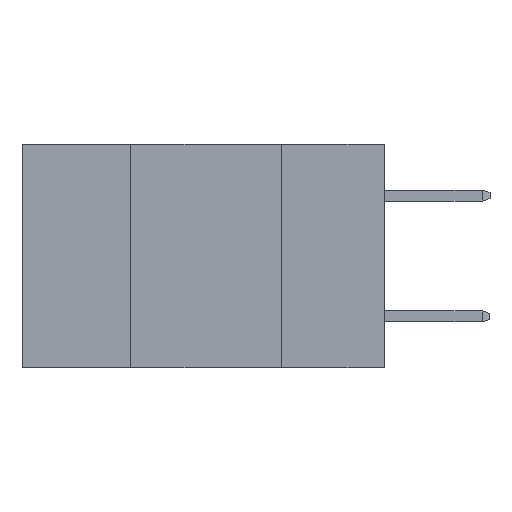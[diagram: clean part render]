
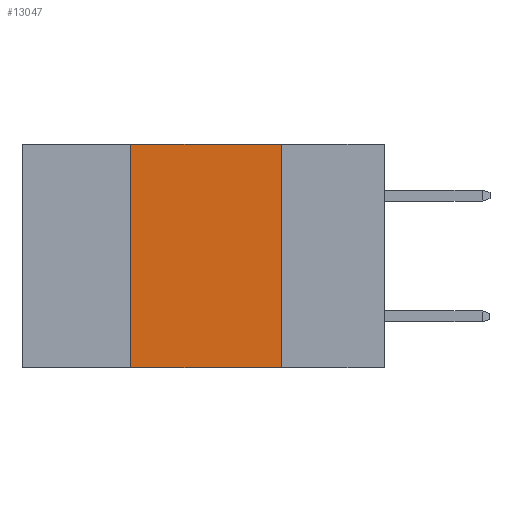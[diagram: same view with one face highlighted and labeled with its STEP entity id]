
A CAD part, left-side view. The second image highlights one B-rep face of the part: STEP entity #13047.
In plain terms, the highlighted planar face has unit normal (-1, 0, 0).
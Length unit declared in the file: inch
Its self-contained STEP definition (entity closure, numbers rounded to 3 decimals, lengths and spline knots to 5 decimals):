
#382 = ORIENTED_EDGE ( 'NONE', *, *, #14201, .F. ) ;
#405 = PLANE ( 'NONE',  #20752 ) ;
#1779 = LINE ( 'NONE', #5530, #19196 ) ;
#3850 = DIRECTION ( 'NONE',  ( 0., 0., -1. ) ) ;
#5530 = CARTESIAN_POINT ( 'NONE',  ( 0., 0.6, 0. ) ) ;
#5657 = CARTESIAN_POINT ( 'NONE',  ( 0., 0.17, 0. ) ) ;
#6548 = CARTESIAN_POINT ( 'NONE',  ( 0., 0.42, -0.37 ) ) ;
#6763 = CARTESIAN_POINT ( 'NONE',  ( 0., 0.6, -0.37 ) ) ;
#6815 = DIRECTION ( 'NONE',  ( 0., -1., 0. ) ) ;
#8472 = VECTOR ( 'NONE', #6815, 39.37008 ) ;
#9575 = VERTEX_POINT ( 'NONE', #10804 ) ;
#9825 = EDGE_CURVE ( 'NONE', #13424, #9575, #12396, .T. ) ;
#10617 = VECTOR ( 'NONE', #17143, 39.37008 ) ;
#10804 = CARTESIAN_POINT ( 'NONE',  ( 0., 0.17, -0.37 ) ) ;
#11161 = FACE_OUTER_BOUND ( 'NONE', #16405, .T. ) ;
#12193 = ORIENTED_EDGE ( 'NONE', *, *, #9825, .T. ) ;
#12254 = CARTESIAN_POINT ( 'NONE',  ( 0., 0.6, 0. ) ) ;
#12290 = DIRECTION ( 'NONE',  ( 0., -1., 0. ) ) ;
#12396 = LINE ( 'NONE', #6763, #8472 ) ;
#12412 = DIRECTION ( 'NONE',  ( 0., 0., -1. ) ) ;
#12538 = VERTEX_POINT ( 'NONE', #12665 ) ;
#12665 = CARTESIAN_POINT ( 'NONE',  ( 0., 0.17, 0. ) ) ;
#13047 = ADVANCED_FACE ( 'NONE', ( #11161 ), #405, .F. ) ;
#13198 = VECTOR ( 'NONE', #12412, 39.37008 ) ;
#13424 = VERTEX_POINT ( 'NONE', #6548 ) ;
#13959 = DIRECTION ( 'NONE',  ( 1., 0., 0. ) ) ;
#14201 = EDGE_CURVE ( 'NONE', #13424, #15941, #19529, .T. ) ;
#14450 = ORIENTED_EDGE ( 'NONE', *, *, #19394, .F. ) ;
#14996 = EDGE_CURVE ( 'NONE', #12538, #9575, #17122, .T. ) ;
#15478 = CARTESIAN_POINT ( 'NONE',  ( 0., 0.42, 0. ) ) ;
#15941 = VERTEX_POINT ( 'NONE', #19726 ) ;
#16405 = EDGE_LOOP ( 'NONE', ( #21201, #14450, #382, #12193 ) ) ;
#17122 = LINE ( 'NONE', #5657, #13198 ) ;
#17143 = DIRECTION ( 'NONE',  ( 0., 0., 1. ) ) ;
#19196 = VECTOR ( 'NONE', #12290, 39.37008 ) ;
#19394 = EDGE_CURVE ( 'NONE', #15941, #12538, #1779, .T. ) ;
#19529 = LINE ( 'NONE', #15478, #10617 ) ;
#19726 = CARTESIAN_POINT ( 'NONE',  ( 0., 0.42, 0. ) ) ;
#20752 = AXIS2_PLACEMENT_3D ( 'NONE', #12254, #13959, #3850 ) ;
#21201 = ORIENTED_EDGE ( 'NONE', *, *, #14996, .F. ) ;
